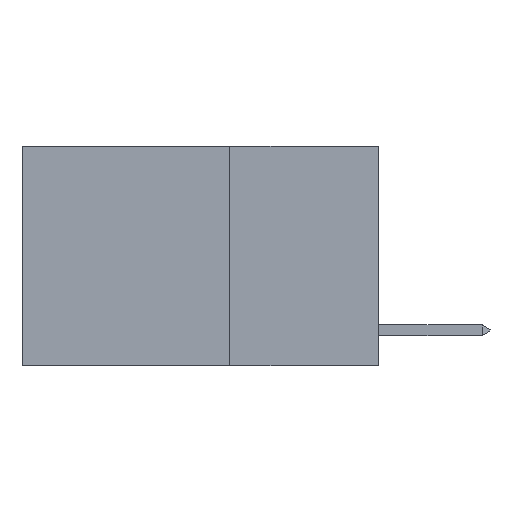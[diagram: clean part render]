
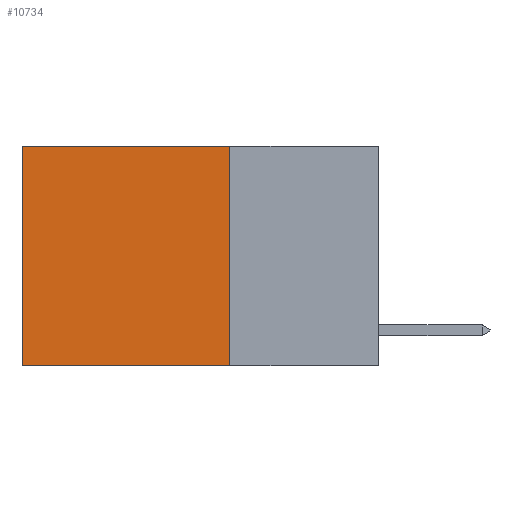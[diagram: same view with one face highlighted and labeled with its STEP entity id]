
A CAD part, left-side view. The second image highlights one B-rep face of the part: STEP entity #10734.
In plain terms, the highlighted planar face has unit normal (-1, 0, 0).
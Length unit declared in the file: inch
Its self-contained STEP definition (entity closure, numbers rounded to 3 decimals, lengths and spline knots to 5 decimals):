
#171 = LINE ( 'NONE', #13432, #8681 ) ;
#492 = VERTEX_POINT ( 'NONE', #12604 ) ;
#645 = EDGE_CURVE ( 'NONE', #10771, #492, #3290, .T. ) ;
#936 = DIRECTION ( 'NONE',  ( 1., 0., 0. ) ) ;
#1090 = EDGE_CURVE ( 'NONE', #8859, #12092, #171, .T. ) ;
#1416 = VECTOR ( 'NONE', #13742, 39.37008 ) ;
#1493 = CARTESIAN_POINT ( 'NONE',  ( 0.2625, 0.25, 0. ) ) ;
#1594 = EDGE_LOOP ( 'NONE', ( #4923, #9000, #4720, #4318 ) ) ;
#2134 = DIRECTION ( 'NONE',  ( 0., 0., -1. ) ) ;
#2686 = VECTOR ( 'NONE', #14278, 39.37008 ) ;
#2717 = CARTESIAN_POINT ( 'NONE',  ( 0.2625, 0.25, 0. ) ) ;
#2742 = CARTESIAN_POINT ( 'NONE',  ( 0.2625, 0.25, -0.37 ) ) ;
#3015 = FACE_OUTER_BOUND ( 'NONE', #1594, .T. ) ;
#3290 = LINE ( 'NONE', #2717, #4159 ) ;
#4159 = VECTOR ( 'NONE', #12077, 39.37008 ) ;
#4162 = LINE ( 'NONE', #9712, #1416 ) ;
#4318 = ORIENTED_EDGE ( 'NONE', *, *, #645, .T. ) ;
#4720 = ORIENTED_EDGE ( 'NONE', *, *, #9078, .F. ) ;
#4923 = ORIENTED_EDGE ( 'NONE', *, *, #5750, .T. ) ;
#5750 = EDGE_CURVE ( 'NONE', #492, #12092, #4162, .T. ) ;
#6414 = DIRECTION ( 'NONE',  ( 0., 1., 0. ) ) ;
#6850 = CARTESIAN_POINT ( 'NONE',  ( 0.2625, 0.25, 0. ) ) ;
#7866 = CARTESIAN_POINT ( 'NONE',  ( 0.2625, 0.25, 0. ) ) ;
#8681 = VECTOR ( 'NONE', #6414, 39.37008 ) ;
#8859 = VERTEX_POINT ( 'NONE', #2742 ) ;
#9000 = ORIENTED_EDGE ( 'NONE', *, *, #1090, .F. ) ;
#9078 = EDGE_CURVE ( 'NONE', #10771, #8859, #14678, .T. ) ;
#9712 = CARTESIAN_POINT ( 'NONE',  ( 0.2625, 0.6, 0. ) ) ;
#10734 = ADVANCED_FACE ( 'NONE', ( #3015 ), #13666, .F. ) ;
#10771 = VERTEX_POINT ( 'NONE', #6850 ) ;
#12077 = DIRECTION ( 'NONE',  ( 0., 1., 0. ) ) ;
#12092 = VERTEX_POINT ( 'NONE', #13238 ) ;
#12604 = CARTESIAN_POINT ( 'NONE',  ( 0.2625, 0.6, 0. ) ) ;
#13238 = CARTESIAN_POINT ( 'NONE',  ( 0.2625, 0.6, -0.37 ) ) ;
#13423 = AXIS2_PLACEMENT_3D ( 'NONE', #7866, #936, #2134 ) ;
#13432 = CARTESIAN_POINT ( 'NONE',  ( 0.2625, 0.25, -0.37 ) ) ;
#13666 = PLANE ( 'NONE',  #13423 ) ;
#13742 = DIRECTION ( 'NONE',  ( 0., 0., -1. ) ) ;
#14278 = DIRECTION ( 'NONE',  ( 0., 0., -1. ) ) ;
#14678 = LINE ( 'NONE', #1493, #2686 ) ;
